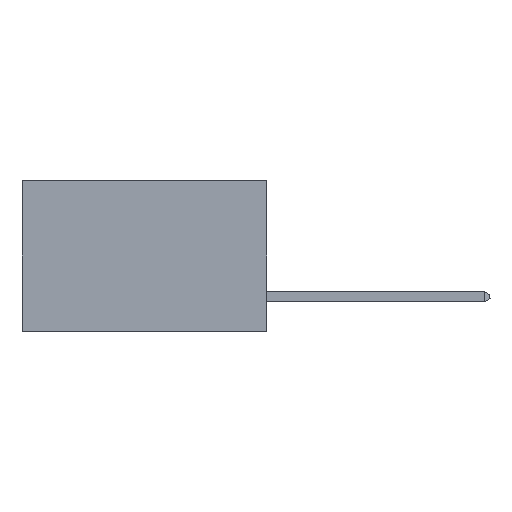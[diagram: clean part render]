
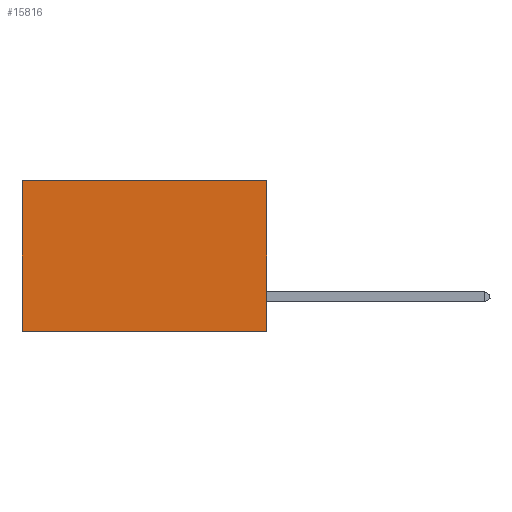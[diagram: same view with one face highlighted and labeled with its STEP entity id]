
A CAD part, left-side view. The second image highlights one B-rep face of the part: STEP entity #15816.
In plain terms, the highlighted planar face has unit normal (-1, 0, 0).
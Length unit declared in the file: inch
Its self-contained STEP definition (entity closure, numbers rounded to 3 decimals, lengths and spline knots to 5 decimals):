
#424 = LINE ( 'NONE', #43948, #16430 ) ;
#4602 = VERTEX_POINT ( 'NONE', #5788 ) ;
#5533 = VECTOR ( 'NONE', #7447, 39.37008 ) ;
#5788 = CARTESIAN_POINT ( 'NONE',  ( 0.2875, 0.6, -0.37 ) ) ;
#7294 = ORIENTED_EDGE ( 'NONE', *, *, #27731, .F. ) ;
#7447 = DIRECTION ( 'NONE',  ( 0., 1., 0. ) ) ;
#9029 = ORIENTED_EDGE ( 'NONE', *, *, #44512, .F. ) ;
#9295 = ORIENTED_EDGE ( 'NONE', *, *, #41682, .T. ) ;
#15398 = EDGE_CURVE ( 'NONE', #28308, #4602, #48310, .T. ) ;
#15487 = VECTOR ( 'NONE', #29117, 39.37008 ) ;
#15816 = ADVANCED_FACE ( 'NONE', ( #22687 ), #27373, .F. ) ;
#16102 = LINE ( 'NONE', #17872, #47759 ) ;
#16430 = VECTOR ( 'NONE', #40312, 39.37008 ) ;
#17872 = CARTESIAN_POINT ( 'NONE',  ( 0.2875, 0., 0. ) ) ;
#18735 = VERTEX_POINT ( 'NONE', #33625 ) ;
#21028 = CARTESIAN_POINT ( 'NONE',  ( 0.2875, 0.6, 0. ) ) ;
#21900 = DIRECTION ( 'NONE',  ( 0., 0., -1. ) ) ;
#22687 = FACE_OUTER_BOUND ( 'NONE', #48567, .T. ) ;
#24567 = CARTESIAN_POINT ( 'NONE',  ( 0.2875, 0.6, 0. ) ) ;
#24743 = CARTESIAN_POINT ( 'NONE',  ( 0.2875, 0., -0.37 ) ) ;
#27373 = PLANE ( 'NONE',  #45373 ) ;
#27731 = EDGE_CURVE ( 'NONE', #18735, #40425, #16102, .T. ) ;
#28308 = VERTEX_POINT ( 'NONE', #24567 ) ;
#29117 = DIRECTION ( 'NONE',  ( 0., 0., -1. ) ) ;
#31691 = CARTESIAN_POINT ( 'NONE',  ( 0.2875, 0., 0. ) ) ;
#33625 = CARTESIAN_POINT ( 'NONE',  ( 0.2875, 0., 0. ) ) ;
#39472 = LINE ( 'NONE', #42127, #5533 ) ;
#40312 = DIRECTION ( 'NONE',  ( 0., 1., 0. ) ) ;
#40425 = VERTEX_POINT ( 'NONE', #24743 ) ;
#41682 = EDGE_CURVE ( 'NONE', #18735, #28308, #424, .T. ) ;
#42127 = CARTESIAN_POINT ( 'NONE',  ( 0.2875, 0., -0.37 ) ) ;
#42918 = DIRECTION ( 'NONE',  ( 1., 0., 0. ) ) ;
#43948 = CARTESIAN_POINT ( 'NONE',  ( 0.2875, 0., 0. ) ) ;
#44512 = EDGE_CURVE ( 'NONE', #40425, #4602, #39472, .T. ) ;
#45373 = AXIS2_PLACEMENT_3D ( 'NONE', #31691, #42918, #46927 ) ;
#45588 = ORIENTED_EDGE ( 'NONE', *, *, #15398, .T. ) ;
#46927 = DIRECTION ( 'NONE',  ( 0., 0., -1. ) ) ;
#47759 = VECTOR ( 'NONE', #21900, 39.37008 ) ;
#48310 = LINE ( 'NONE', #21028, #15487 ) ;
#48567 = EDGE_LOOP ( 'NONE', ( #45588, #9029, #7294, #9295 ) ) ;
